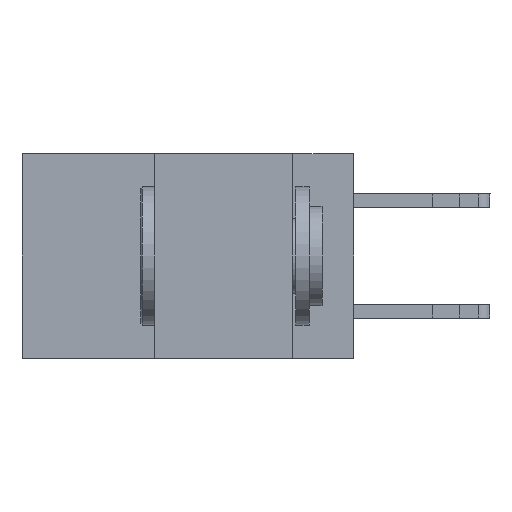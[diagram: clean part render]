
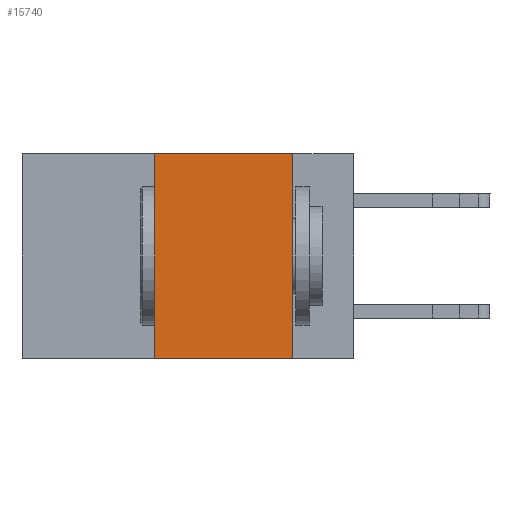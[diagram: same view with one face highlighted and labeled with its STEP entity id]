
A CAD part, left-side view. The second image highlights one B-rep face of the part: STEP entity #15740.
In plain terms, the highlighted planar face has unit normal (-1, 0, 0).
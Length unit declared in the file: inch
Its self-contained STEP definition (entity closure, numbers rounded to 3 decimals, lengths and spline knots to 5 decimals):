
#262 = DIRECTION ( 'NONE',  ( 0., 0., -1. ) ) ;
#351 = AXIS2_PLACEMENT_3D ( 'NONE', #22904, #5269, #20319 ) ;
#369 = VERTEX_POINT ( 'NONE', #16861 ) ;
#2248 = VECTOR ( 'NONE', #262, 39.37008 ) ;
#5269 = DIRECTION ( 'NONE',  ( 1., 0., 0. ) ) ;
#5399 = VERTEX_POINT ( 'NONE', #16597 ) ;
#6968 = CARTESIAN_POINT ( 'NONE',  ( 0., 0.6, -0.37 ) ) ;
#7541 = VERTEX_POINT ( 'NONE', #21310 ) ;
#8336 = PLANE ( 'NONE',  #351 ) ;
#8581 = LINE ( 'NONE', #33181, #21953 ) ;
#9675 = EDGE_CURVE ( 'NONE', #369, #24450, #14973, .T. ) ;
#9884 = EDGE_CURVE ( 'NONE', #5399, #7541, #8581, .T. ) ;
#10097 = ORIENTED_EDGE ( 'NONE', *, *, #9675, .T. ) ;
#12755 = CARTESIAN_POINT ( 'NONE',  ( 0., 0.36, 0. ) ) ;
#14692 = LINE ( 'NONE', #21235, #2248 ) ;
#14970 = EDGE_CURVE ( 'NONE', #369, #5399, #15947, .T. ) ;
#14973 = LINE ( 'NONE', #6968, #16363 ) ;
#15016 = VECTOR ( 'NONE', #33634, 39.37008 ) ;
#15036 = ORIENTED_EDGE ( 'NONE', *, *, #14970, .F. ) ;
#15740 = ADVANCED_FACE ( 'NONE', ( #18473 ), #8336, .F. ) ;
#15947 = LINE ( 'NONE', #12755, #15016 ) ;
#16363 = VECTOR ( 'NONE', #35927, 39.37008 ) ;
#16597 = CARTESIAN_POINT ( 'NONE',  ( 0., 0.36, 0. ) ) ;
#16861 = CARTESIAN_POINT ( 'NONE',  ( 0., 0.36, -0.37 ) ) ;
#18473 = FACE_OUTER_BOUND ( 'NONE', #22156, .T. ) ;
#20319 = DIRECTION ( 'NONE',  ( 0., 0., -1. ) ) ;
#21235 = CARTESIAN_POINT ( 'NONE',  ( 0., 0.11, 0. ) ) ;
#21310 = CARTESIAN_POINT ( 'NONE',  ( 0., 0.11, 0. ) ) ;
#21953 = VECTOR ( 'NONE', #27968, 39.37008 ) ;
#22156 = EDGE_LOOP ( 'NONE', ( #24669, #31039, #15036, #10097 ) ) ;
#22904 = CARTESIAN_POINT ( 'NONE',  ( 0., 0.6, 0. ) ) ;
#24269 = CARTESIAN_POINT ( 'NONE',  ( 0., 0.11, -0.37 ) ) ;
#24450 = VERTEX_POINT ( 'NONE', #24269 ) ;
#24669 = ORIENTED_EDGE ( 'NONE', *, *, #34055, .F. ) ;
#27968 = DIRECTION ( 'NONE',  ( 0., -1., 0. ) ) ;
#31039 = ORIENTED_EDGE ( 'NONE', *, *, #9884, .F. ) ;
#33181 = CARTESIAN_POINT ( 'NONE',  ( 0., 0.6, 0. ) ) ;
#33634 = DIRECTION ( 'NONE',  ( 0., 0., 1. ) ) ;
#34055 = EDGE_CURVE ( 'NONE', #7541, #24450, #14692, .T. ) ;
#35927 = DIRECTION ( 'NONE',  ( 0., -1., 0. ) ) ;
